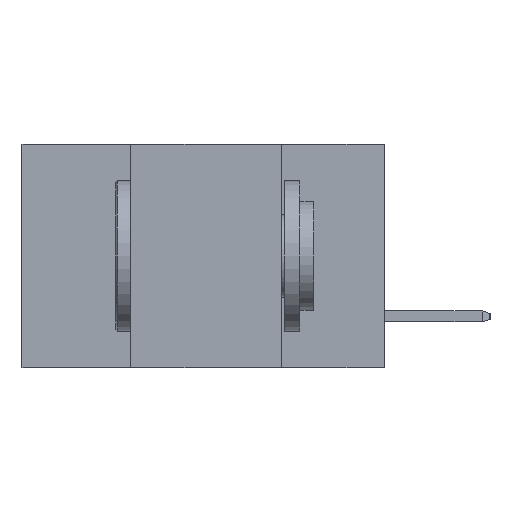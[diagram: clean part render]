
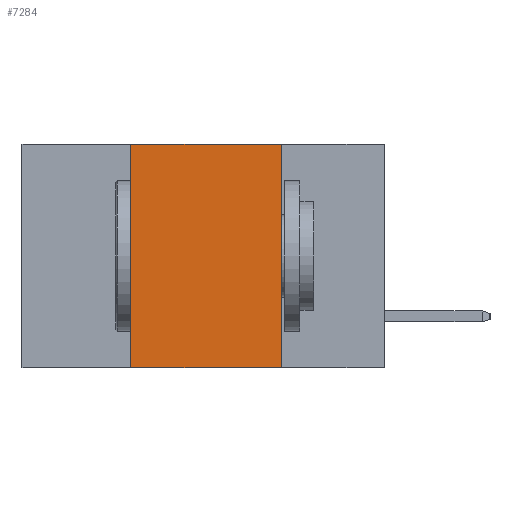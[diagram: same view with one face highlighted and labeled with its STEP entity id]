
A CAD part, left-side view. The second image highlights one B-rep face of the part: STEP entity #7284.
In plain terms, the highlighted planar face has unit normal (-1, 0, 0).
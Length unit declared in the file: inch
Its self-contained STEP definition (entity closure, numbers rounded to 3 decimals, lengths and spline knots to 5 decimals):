
#100 = EDGE_CURVE ( 'NONE', #3327, #1046, #7344, .T. ) ;
#617 = CARTESIAN_POINT ( 'NONE',  ( 0., 0.42, -0.37 ) ) ;
#829 = VERTEX_POINT ( 'NONE', #5729 ) ;
#1046 = VERTEX_POINT ( 'NONE', #2440 ) ;
#1908 = ORIENTED_EDGE ( 'NONE', *, *, #3150, .F. ) ;
#2054 = CARTESIAN_POINT ( 'NONE',  ( 0., 0.6, 0. ) ) ;
#2295 = VERTEX_POINT ( 'NONE', #3019 ) ;
#2440 = CARTESIAN_POINT ( 'NONE',  ( 0., 0.42, 0. ) ) ;
#2604 = ORIENTED_EDGE ( 'NONE', *, *, #100, .F. ) ;
#2954 = DIRECTION ( 'NONE',  ( 0., 0., -1. ) ) ;
#3019 = CARTESIAN_POINT ( 'NONE',  ( 0., 0.17, 0. ) ) ;
#3150 = EDGE_CURVE ( 'NONE', #2295, #829, #6185, .T. ) ;
#3327 = VERTEX_POINT ( 'NONE', #617 ) ;
#3477 = LINE ( 'NONE', #8183, #3754 ) ;
#3754 = VECTOR ( 'NONE', #9039, 39.37008 ) ;
#4516 = CARTESIAN_POINT ( 'NONE',  ( 0., 0.6, -0.37 ) ) ;
#5067 = FACE_OUTER_BOUND ( 'NONE', #5471, .T. ) ;
#5369 = DIRECTION ( 'NONE',  ( 0., -1., 0. ) ) ;
#5471 = EDGE_LOOP ( 'NONE', ( #1908, #11009, #2604, #8481 ) ) ;
#5729 = CARTESIAN_POINT ( 'NONE',  ( 0., 0.17, -0.37 ) ) ;
#6185 = LINE ( 'NONE', #6310, #10718 ) ;
#6310 = CARTESIAN_POINT ( 'NONE',  ( 0., 0.17, 0. ) ) ;
#6331 = PLANE ( 'NONE',  #8694 ) ;
#6490 = CARTESIAN_POINT ( 'NONE',  ( 0., 0.42, 0. ) ) ;
#7284 = ADVANCED_FACE ( 'NONE', ( #5067 ), #6331, .F. ) ;
#7344 = LINE ( 'NONE', #6490, #9056 ) ;
#7580 = VECTOR ( 'NONE', #5369, 39.37008 ) ;
#7835 = LINE ( 'NONE', #4516, #7580 ) ;
#8042 = DIRECTION ( 'NONE',  ( 0., 0., -1. ) ) ;
#8049 = DIRECTION ( 'NONE',  ( 1., 0., 0. ) ) ;
#8183 = CARTESIAN_POINT ( 'NONE',  ( 0., 0.6, 0. ) ) ;
#8481 = ORIENTED_EDGE ( 'NONE', *, *, #8491, .T. ) ;
#8491 = EDGE_CURVE ( 'NONE', #3327, #829, #7835, .T. ) ;
#8694 = AXIS2_PLACEMENT_3D ( 'NONE', #2054, #8049, #2954 ) ;
#9039 = DIRECTION ( 'NONE',  ( 0., -1., 0. ) ) ;
#9056 = VECTOR ( 'NONE', #9574, 39.37008 ) ;
#9574 = DIRECTION ( 'NONE',  ( 0., 0., 1. ) ) ;
#9955 = EDGE_CURVE ( 'NONE', #1046, #2295, #3477, .T. ) ;
#10718 = VECTOR ( 'NONE', #8042, 39.37008 ) ;
#11009 = ORIENTED_EDGE ( 'NONE', *, *, #9955, .F. ) ;
